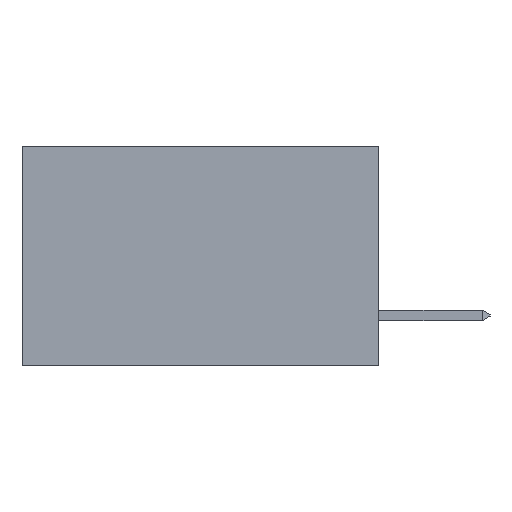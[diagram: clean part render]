
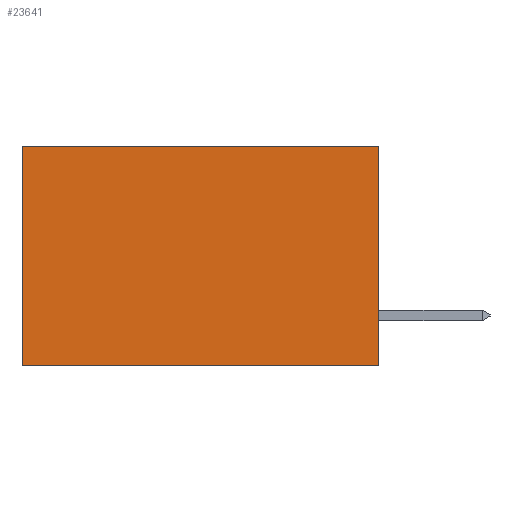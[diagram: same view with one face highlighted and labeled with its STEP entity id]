
A CAD part, left-side view. The second image highlights one B-rep face of the part: STEP entity #23641.
In plain terms, the highlighted planar face has unit normal (-1, 0, 0).
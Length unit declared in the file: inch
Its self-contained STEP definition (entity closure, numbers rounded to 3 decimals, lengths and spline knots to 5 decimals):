
#1363 = CARTESIAN_POINT ( 'NONE',  ( 0.2615, 0., -0.37 ) ) ;
#1492 = CARTESIAN_POINT ( 'NONE',  ( 0.2615, 0., -0.37 ) ) ;
#1500 = CARTESIAN_POINT ( 'NONE',  ( 0.2615, 0.6, -0.37 ) ) ;
#2655 = VECTOR ( 'NONE', #20132, 39.37008 ) ;
#4708 = VERTEX_POINT ( 'NONE', #7627 ) ;
#5068 = VECTOR ( 'NONE', #18639, 39.37008 ) ;
#5584 = CARTESIAN_POINT ( 'NONE',  ( 0.2615, 0., -0.37 ) ) ;
#5699 = AXIS2_PLACEMENT_3D ( 'NONE', #1492, #9097, #22008 ) ;
#6024 = EDGE_CURVE ( 'NONE', #13238, #22078, #14626, .T. ) ;
#6213 = ORIENTED_EDGE ( 'NONE', *, *, #21062, .T. ) ;
#7627 = CARTESIAN_POINT ( 'NONE',  ( 0.2615, 0.6, -0.37 ) ) ;
#9097 = DIRECTION ( 'NONE',  ( 1., 0., 0. ) ) ;
#9627 = VECTOR ( 'NONE', #14888, 39.37008 ) ;
#12585 = ORIENTED_EDGE ( 'NONE', *, *, #6024, .T. ) ;
#12861 = LINE ( 'NONE', #1363, #22027 ) ;
#13216 = VERTEX_POINT ( 'NONE', #22156 ) ;
#13238 = VERTEX_POINT ( 'NONE', #16779 ) ;
#14521 = ORIENTED_EDGE ( 'NONE', *, *, #17757, .F. ) ;
#14626 = LINE ( 'NONE', #15359, #9627 ) ;
#14746 = FACE_OUTER_BOUND ( 'NONE', #17372, .T. ) ;
#14888 = DIRECTION ( 'NONE',  ( 0., 1., 0. ) ) ;
#15359 = CARTESIAN_POINT ( 'NONE',  ( 0.2615, 0., 0. ) ) ;
#16779 = CARTESIAN_POINT ( 'NONE',  ( 0.2615, 0., 0. ) ) ;
#17372 = EDGE_LOOP ( 'NONE', ( #6213, #23916, #14521, #12585 ) ) ;
#17607 = LINE ( 'NONE', #1500, #2655 ) ;
#17757 = EDGE_CURVE ( 'NONE', #13238, #13216, #12861, .T. ) ;
#18380 = PLANE ( 'NONE',  #5699 ) ;
#18639 = DIRECTION ( 'NONE',  ( 0., 1., 0. ) ) ;
#19356 = CARTESIAN_POINT ( 'NONE',  ( 0.2615, 0.6, 0. ) ) ;
#19363 = LINE ( 'NONE', #5584, #5068 ) ;
#19697 = EDGE_CURVE ( 'NONE', #13216, #4708, #19363, .T. ) ;
#20132 = DIRECTION ( 'NONE',  ( 0., 0., -1. ) ) ;
#21062 = EDGE_CURVE ( 'NONE', #22078, #4708, #17607, .T. ) ;
#21810 = DIRECTION ( 'NONE',  ( 0., 0., -1. ) ) ;
#22008 = DIRECTION ( 'NONE',  ( 0., 0., -1. ) ) ;
#22027 = VECTOR ( 'NONE', #21810, 39.37008 ) ;
#22078 = VERTEX_POINT ( 'NONE', #19356 ) ;
#22156 = CARTESIAN_POINT ( 'NONE',  ( 0.2615, 0., -0.37 ) ) ;
#23641 = ADVANCED_FACE ( 'NONE', ( #14746 ), #18380, .F. ) ;
#23916 = ORIENTED_EDGE ( 'NONE', *, *, #19697, .F. ) ;
